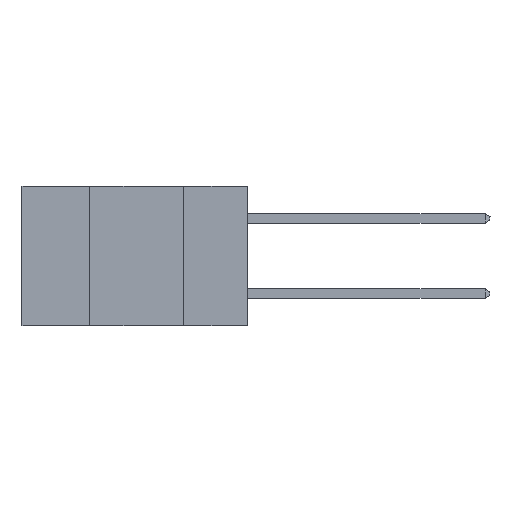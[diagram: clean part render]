
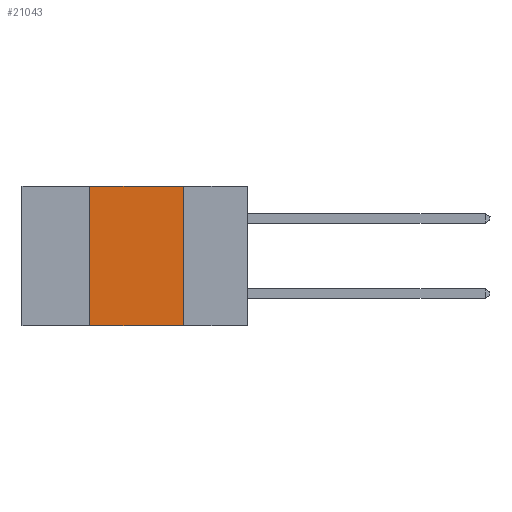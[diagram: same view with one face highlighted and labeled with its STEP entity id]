
A CAD part, left-side view. The second image highlights one B-rep face of the part: STEP entity #21043.
In plain terms, the highlighted planar face has unit normal (-1, 0, 0).
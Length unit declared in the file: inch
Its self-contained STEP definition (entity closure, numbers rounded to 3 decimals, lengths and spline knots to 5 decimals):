
#2066 = ORIENTED_EDGE ( 'NONE', *, *, #8476, .T. ) ;
#3176 = VERTEX_POINT ( 'NONE', #26551 ) ;
#5341 = VECTOR ( 'NONE', #7541, 39.37008 ) ;
#5980 = EDGE_LOOP ( 'NONE', ( #23068, #18879, #13675, #2066 ) ) ;
#6172 = LINE ( 'NONE', #11113, #5341 ) ;
#6790 = EDGE_CURVE ( 'NONE', #11206, #9666, #18968, .T. ) ;
#7463 = VERTEX_POINT ( 'NONE', #8379 ) ;
#7541 = DIRECTION ( 'NONE',  ( 0., -1., 0. ) ) ;
#8379 = CARTESIAN_POINT ( 'NONE',  ( 0., 0.17, 0. ) ) ;
#8476 = EDGE_CURVE ( 'NONE', #11206, #3176, #6172, .T. ) ;
#8812 = VECTOR ( 'NONE', #25345, 39.37008 ) ;
#8873 = AXIS2_PLACEMENT_3D ( 'NONE', #11574, #28984, #14101 ) ;
#9666 = VERTEX_POINT ( 'NONE', #29962 ) ;
#10878 = CARTESIAN_POINT ( 'NONE',  ( 0., 0.42, -0.37 ) ) ;
#11113 = CARTESIAN_POINT ( 'NONE',  ( 0., 0.6, -0.37 ) ) ;
#11206 = VERTEX_POINT ( 'NONE', #10878 ) ;
#11276 = CARTESIAN_POINT ( 'NONE',  ( 0., 0.42, 0. ) ) ;
#11574 = CARTESIAN_POINT ( 'NONE',  ( 0., 0.6, 0. ) ) ;
#13393 = EDGE_CURVE ( 'NONE', #9666, #7463, #30106, .T. ) ;
#13675 = ORIENTED_EDGE ( 'NONE', *, *, #6790, .F. ) ;
#14101 = DIRECTION ( 'NONE',  ( 0., 0., -1. ) ) ;
#16618 = CARTESIAN_POINT ( 'NONE',  ( 0., 0.6, 0. ) ) ;
#16964 = VECTOR ( 'NONE', #19106, 39.37008 ) ;
#17004 = EDGE_CURVE ( 'NONE', #7463, #3176, #28735, .T. ) ;
#18187 = VECTOR ( 'NONE', #24726, 39.37008 ) ;
#18879 = ORIENTED_EDGE ( 'NONE', *, *, #13393, .F. ) ;
#18968 = LINE ( 'NONE', #11276, #18187 ) ;
#19106 = DIRECTION ( 'NONE',  ( 0., -1., 0. ) ) ;
#21043 = ADVANCED_FACE ( 'NONE', ( #24409 ), #26484, .F. ) ;
#22885 = CARTESIAN_POINT ( 'NONE',  ( 0., 0.17, 0. ) ) ;
#23068 = ORIENTED_EDGE ( 'NONE', *, *, #17004, .F. ) ;
#24409 = FACE_OUTER_BOUND ( 'NONE', #5980, .T. ) ;
#24726 = DIRECTION ( 'NONE',  ( 0., 0., 1. ) ) ;
#25345 = DIRECTION ( 'NONE',  ( 0., 0., -1. ) ) ;
#26484 = PLANE ( 'NONE',  #8873 ) ;
#26551 = CARTESIAN_POINT ( 'NONE',  ( 0., 0.17, -0.37 ) ) ;
#28735 = LINE ( 'NONE', #22885, #8812 ) ;
#28984 = DIRECTION ( 'NONE',  ( 1., 0., 0. ) ) ;
#29962 = CARTESIAN_POINT ( 'NONE',  ( 0., 0.42, 0. ) ) ;
#30106 = LINE ( 'NONE', #16618, #16964 ) ;
